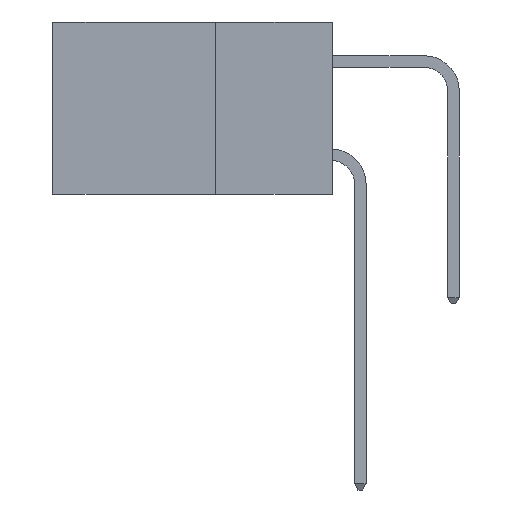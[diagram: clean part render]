
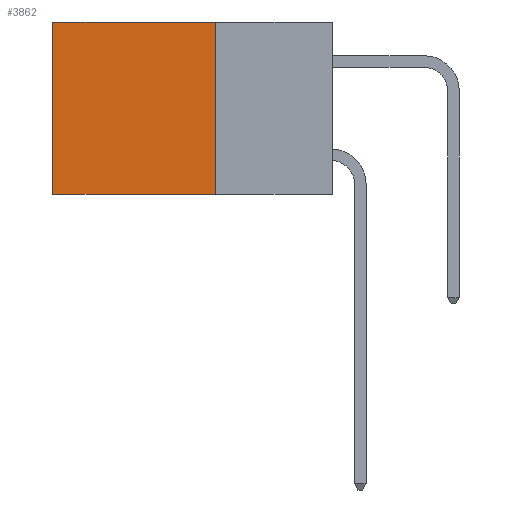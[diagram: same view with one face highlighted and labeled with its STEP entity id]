
A CAD part, left-side view. The second image highlights one B-rep face of the part: STEP entity #3862.
In plain terms, the highlighted planar face has unit normal (-1, 0, 0).
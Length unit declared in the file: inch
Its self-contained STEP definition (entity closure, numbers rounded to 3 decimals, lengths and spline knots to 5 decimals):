
#761 = VECTOR ( 'NONE', #3772, 39.37008 ) ;
#871 = CARTESIAN_POINT ( 'NONE',  ( 0.2615, 0.25, -0.37 ) ) ;
#880 = CARTESIAN_POINT ( 'NONE',  ( 0.2615, 0.25, 0. ) ) ;
#1379 = VERTEX_POINT ( 'NONE', #7903 ) ;
#2218 = ORIENTED_EDGE ( 'NONE', *, *, #8130, .T. ) ;
#2253 = VERTEX_POINT ( 'NONE', #9356 ) ;
#2911 = CARTESIAN_POINT ( 'NONE',  ( 0.2615, 0.6, -0.37 ) ) ;
#3047 = EDGE_CURVE ( 'NONE', #15598, #2253, #7305, .T. ) ;
#3124 = CARTESIAN_POINT ( 'NONE',  ( 0.2615, 0.25, 0. ) ) ;
#3180 = CARTESIAN_POINT ( 'NONE',  ( 0.2615, 0.25, -0.37 ) ) ;
#3187 = LINE ( 'NONE', #2911, #5662 ) ;
#3459 = LINE ( 'NONE', #871, #14745 ) ;
#3472 = VECTOR ( 'NONE', #4634, 39.37008 ) ;
#3772 = DIRECTION ( 'NONE',  ( 0., 1., 0. ) ) ;
#3862 = ADVANCED_FACE ( 'NONE', ( #9150 ), #7405, .F. ) ;
#4172 = DIRECTION ( 'NONE',  ( 0., 0., -1. ) ) ;
#4253 = LINE ( 'NONE', #880, #3472 ) ;
#4270 = CARTESIAN_POINT ( 'NONE',  ( 0.2615, 0.25, -0.37 ) ) ;
#4634 = DIRECTION ( 'NONE',  ( 0., 1., 0. ) ) ;
#5160 = EDGE_CURVE ( 'NONE', #15572, #1379, #4253, .T. ) ;
#5662 = VECTOR ( 'NONE', #4172, 39.37008 ) ;
#5696 = EDGE_CURVE ( 'NONE', #15572, #15598, #3459, .T. ) ;
#6277 = EDGE_LOOP ( 'NONE', ( #2218, #7014, #9652, #8696 ) ) ;
#7014 = ORIENTED_EDGE ( 'NONE', *, *, #3047, .F. ) ;
#7243 = DIRECTION ( 'NONE',  ( 0., 0., -1. ) ) ;
#7262 = DIRECTION ( 'NONE',  ( 1., 0., 0. ) ) ;
#7282 = CARTESIAN_POINT ( 'NONE',  ( 0.2615, 0.25, -0.37 ) ) ;
#7305 = LINE ( 'NONE', #4270, #761 ) ;
#7405 = PLANE ( 'NONE',  #15373 ) ;
#7903 = CARTESIAN_POINT ( 'NONE',  ( 0.2615, 0.6, 0. ) ) ;
#8012 = DIRECTION ( 'NONE',  ( 0., 0., -1. ) ) ;
#8130 = EDGE_CURVE ( 'NONE', #1379, #2253, #3187, .T. ) ;
#8696 = ORIENTED_EDGE ( 'NONE', *, *, #5160, .T. ) ;
#9150 = FACE_OUTER_BOUND ( 'NONE', #6277, .T. ) ;
#9356 = CARTESIAN_POINT ( 'NONE',  ( 0.2615, 0.6, -0.37 ) ) ;
#9652 = ORIENTED_EDGE ( 'NONE', *, *, #5696, .F. ) ;
#14745 = VECTOR ( 'NONE', #8012, 39.37008 ) ;
#15373 = AXIS2_PLACEMENT_3D ( 'NONE', #7282, #7262, #7243 ) ;
#15572 = VERTEX_POINT ( 'NONE', #3124 ) ;
#15598 = VERTEX_POINT ( 'NONE', #3180 ) ;
